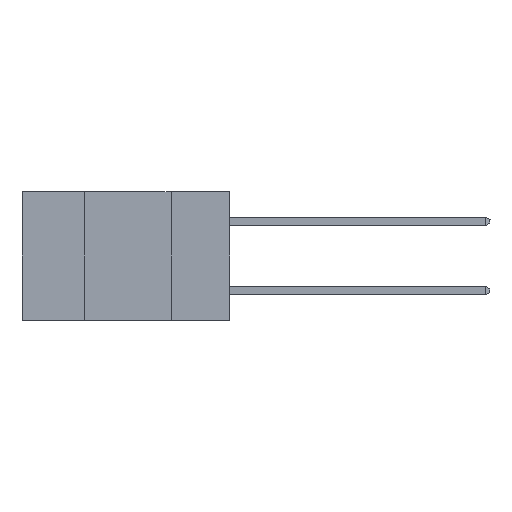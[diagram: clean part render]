
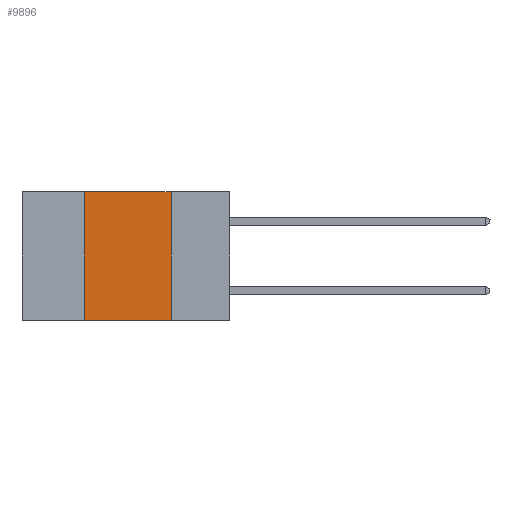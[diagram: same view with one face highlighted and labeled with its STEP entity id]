
A CAD part, left-side view. The second image highlights one B-rep face of the part: STEP entity #9896.
In plain terms, the highlighted planar face has unit normal (-1, 0, 0).
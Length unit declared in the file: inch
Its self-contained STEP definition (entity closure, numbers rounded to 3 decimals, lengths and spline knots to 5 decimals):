
#725 = EDGE_LOOP ( 'NONE', ( #21627, #22667, #7893, #7692 ) ) ;
#1254 = VERTEX_POINT ( 'NONE', #17456 ) ;
#1373 = CARTESIAN_POINT ( 'NONE',  ( 0., 0.6, 0. ) ) ;
#1876 = CARTESIAN_POINT ( 'NONE',  ( 0., 0.6, 0. ) ) ;
#1952 = DIRECTION ( 'NONE',  ( 0., -1., 0. ) ) ;
#3292 = EDGE_CURVE ( 'NONE', #11026, #1254, #11428, .T. ) ;
#5648 = EDGE_CURVE ( 'NONE', #17433, #11026, #7787, .T. ) ;
#6229 = VECTOR ( 'NONE', #20957, 39.37008 ) ;
#6427 = CARTESIAN_POINT ( 'NONE',  ( 0., 0.17, 0. ) ) ;
#6839 = CARTESIAN_POINT ( 'NONE',  ( 0., 0.6, -0.37 ) ) ;
#7275 = DIRECTION ( 'NONE',  ( 1., 0., 0. ) ) ;
#7692 = ORIENTED_EDGE ( 'NONE', *, *, #24067, .T. ) ;
#7787 = LINE ( 'NONE', #1876, #12870 ) ;
#7893 = ORIENTED_EDGE ( 'NONE', *, *, #21101, .F. ) ;
#9896 = ADVANCED_FACE ( 'NONE', ( #16445 ), #17613, .F. ) ;
#10318 = LINE ( 'NONE', #18846, #6229 ) ;
#11026 = VERTEX_POINT ( 'NONE', #22146 ) ;
#11428 = LINE ( 'NONE', #6427, #19314 ) ;
#12870 = VECTOR ( 'NONE', #1952, 39.37008 ) ;
#13254 = CARTESIAN_POINT ( 'NONE',  ( 0., 0.42, -0.37 ) ) ;
#15542 = CARTESIAN_POINT ( 'NONE',  ( 0., 0.42, 0. ) ) ;
#16445 = FACE_OUTER_BOUND ( 'NONE', #725, .T. ) ;
#17433 = VERTEX_POINT ( 'NONE', #15542 ) ;
#17456 = CARTESIAN_POINT ( 'NONE',  ( 0., 0.17, -0.37 ) ) ;
#17613 = PLANE ( 'NONE',  #22578 ) ;
#18341 = LINE ( 'NONE', #6839, #20548 ) ;
#18846 = CARTESIAN_POINT ( 'NONE',  ( 0., 0.42, 0. ) ) ;
#19060 = VERTEX_POINT ( 'NONE', #13254 ) ;
#19314 = VECTOR ( 'NONE', #20539, 39.37008 ) ;
#19626 = DIRECTION ( 'NONE',  ( 0., -1., 0. ) ) ;
#20539 = DIRECTION ( 'NONE',  ( 0., 0., -1. ) ) ;
#20548 = VECTOR ( 'NONE', #19626, 39.37008 ) ;
#20957 = DIRECTION ( 'NONE',  ( 0., 0., 1. ) ) ;
#21101 = EDGE_CURVE ( 'NONE', #19060, #17433, #10318, .T. ) ;
#21397 = DIRECTION ( 'NONE',  ( 0., 0., -1. ) ) ;
#21627 = ORIENTED_EDGE ( 'NONE', *, *, #3292, .F. ) ;
#22146 = CARTESIAN_POINT ( 'NONE',  ( 0., 0.17, 0. ) ) ;
#22578 = AXIS2_PLACEMENT_3D ( 'NONE', #1373, #7275, #21397 ) ;
#22667 = ORIENTED_EDGE ( 'NONE', *, *, #5648, .F. ) ;
#24067 = EDGE_CURVE ( 'NONE', #19060, #1254, #18341, .T. ) ;
